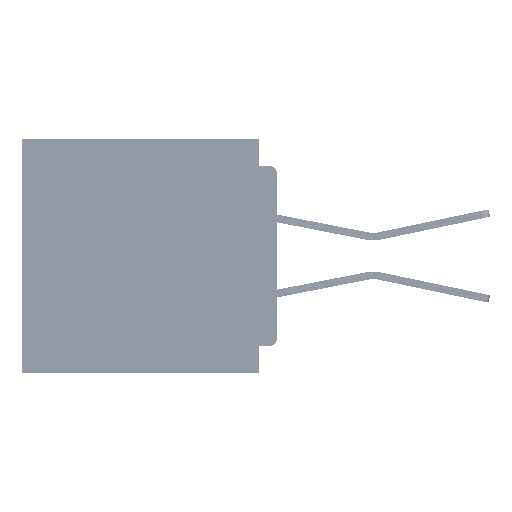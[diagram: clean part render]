
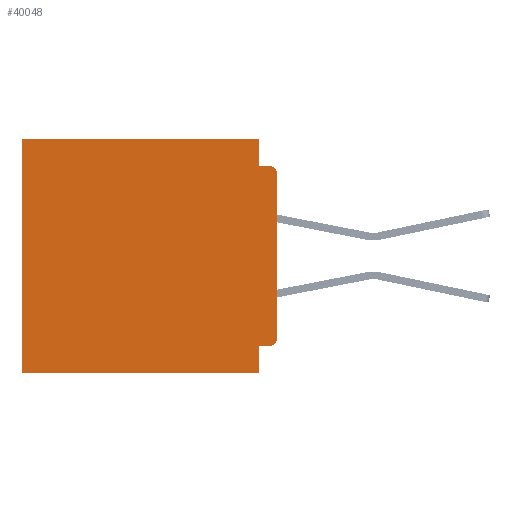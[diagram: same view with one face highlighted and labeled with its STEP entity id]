
A CAD part, left-side view. The second image highlights one B-rep face of the part: STEP entity #40048.
In plain terms, the highlighted planar face has unit normal (-1, 0, 0).
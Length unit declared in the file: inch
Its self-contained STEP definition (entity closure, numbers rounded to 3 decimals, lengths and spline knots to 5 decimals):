
#981 = VERTEX_POINT ( 'NONE', #3065 ) ;
#1917 = DIRECTION ( 'NONE',  ( 0., 1., 0. ) ) ;
#1973 = CARTESIAN_POINT ( 'NONE',  ( 0.3, 0.015, -0.34 ) ) ;
#2078 = ORIENTED_EDGE ( 'NONE', *, *, #9908, .T. ) ;
#2806 = VERTEX_POINT ( 'NONE', #18349 ) ;
#3065 = CARTESIAN_POINT ( 'NONE',  ( 0.3, 0.031, -0.045 ) ) ;
#3444 = EDGE_CURVE ( 'NONE', #34195, #33363, #9608, .T. ) ;
#4538 = CARTESIAN_POINT ( 'NONE',  ( 0.3, 0., -0.355 ) ) ;
#4986 = PLANE ( 'NONE',  #46262 ) ;
#5050 = CARTESIAN_POINT ( 'NONE',  ( 0.3, 0., -0.34 ) ) ;
#5322 = EDGE_CURVE ( 'NONE', #2806, #43426, #53814, .T. ) ;
#5660 = EDGE_CURVE ( 'NONE', #49036, #11780, #35707, .T. ) ;
#7135 = DIRECTION ( 'NONE',  ( 0., 0., -1. ) ) ;
#7487 = CARTESIAN_POINT ( 'NONE',  ( 0.3, 0.015, -0.06 ) ) ;
#8285 = ORIENTED_EDGE ( 'NONE', *, *, #41139, .T. ) ;
#8566 = VERTEX_POINT ( 'NONE', #5050 ) ;
#8852 = LINE ( 'NONE', #54566, #10474 ) ;
#8932 = EDGE_LOOP ( 'NONE', ( #15357, #13591, #13885, #32262, #8285, #56906, #37852, #56717, #35630, #2078 ) ) ;
#9608 = LINE ( 'NONE', #4538, #35096 ) ;
#9908 = EDGE_CURVE ( 'NONE', #34195, #8566, #17360, .T. ) ;
#10119 = CARTESIAN_POINT ( 'NONE',  ( 0.3, 0., -0.4 ) ) ;
#10474 = VECTOR ( 'NONE', #19109, 39.37008 ) ;
#10681 = CARTESIAN_POINT ( 'NONE',  ( 0.3, 0., -0.4 ) ) ;
#11780 = VERTEX_POINT ( 'NONE', #47954 ) ;
#12627 = DIRECTION ( 'NONE',  ( 0., 0., -1. ) ) ;
#13591 = ORIENTED_EDGE ( 'NONE', *, *, #5322, .T. ) ;
#13675 = VECTOR ( 'NONE', #29118, 39.37008 ) ;
#13885 = ORIENTED_EDGE ( 'NONE', *, *, #42511, .F. ) ;
#15235 = DIRECTION ( 'NONE',  ( 1., 0., 0. ) ) ;
#15357 = ORIENTED_EDGE ( 'NONE', *, *, #38884, .F. ) ;
#15817 = DIRECTION ( 'NONE',  ( 0., 0., -1. ) ) ;
#16157 = CARTESIAN_POINT ( 'NONE',  ( 0.3, 0.437, -0.4 ) ) ;
#17360 = CIRCLE ( 'NONE', #58397, 0.015 ) ;
#18349 = CARTESIAN_POINT ( 'NONE',  ( 0.3, 0., -0.06 ) ) ;
#19109 = DIRECTION ( 'NONE',  ( 0., 1., 0. ) ) ;
#20151 = CARTESIAN_POINT ( 'NONE',  ( 0.3, 0., -0.4 ) ) ;
#20365 = DIRECTION ( 'NONE',  ( 0., 0., -1. ) ) ;
#21446 = CARTESIAN_POINT ( 'NONE',  ( 0.3, 0.031, -0.355 ) ) ;
#21928 = CARTESIAN_POINT ( 'NONE',  ( 0.3, 0.015, -0.045 ) ) ;
#22177 = VECTOR ( 'NONE', #60693, 39.37008 ) ;
#24270 = DIRECTION ( 'NONE',  ( 0., -1., 0. ) ) ;
#24896 = CARTESIAN_POINT ( 'NONE',  ( 0.3, 0.031, -0.4 ) ) ;
#28815 = LINE ( 'NONE', #64538, #13675 ) ;
#28923 = AXIS2_PLACEMENT_3D ( 'NONE', #7487, #43062, #12627 ) ;
#29118 = DIRECTION ( 'NONE',  ( 0., 0., -1. ) ) ;
#32262 = ORIENTED_EDGE ( 'NONE', *, *, #35879, .F. ) ;
#33363 = VERTEX_POINT ( 'NONE', #21446 ) ;
#34195 = VERTEX_POINT ( 'NONE', #64536 ) ;
#34668 = VECTOR ( 'NONE', #15817, 39.37008 ) ;
#35096 = VECTOR ( 'NONE', #1917, 39.37008 ) ;
#35630 = ORIENTED_EDGE ( 'NONE', *, *, #3444, .F. ) ;
#35707 = LINE ( 'NONE', #20151, #22177 ) ;
#35879 = EDGE_CURVE ( 'NONE', #44845, #981, #36680, .T. ) ;
#36680 = LINE ( 'NONE', #60914, #46906 ) ;
#37616 = DIRECTION ( 'NONE',  ( -1., 0., 0. ) ) ;
#37772 = VECTOR ( 'NONE', #56708, 39.37008 ) ;
#37852 = ORIENTED_EDGE ( 'NONE', *, *, #5660, .F. ) ;
#38531 = FACE_OUTER_BOUND ( 'NONE', #8932, .T. ) ;
#38884 = EDGE_CURVE ( 'NONE', #2806, #8566, #48095, .T. ) ;
#40048 = ADVANCED_FACE ( 'NONE', ( #38531 ), #4986, .F. ) ;
#40275 = CARTESIAN_POINT ( 'NONE',  ( 0.3, 0.031, 0. ) ) ;
#41139 = EDGE_CURVE ( 'NONE', #44845, #52347, #8852, .T. ) ;
#42511 = EDGE_CURVE ( 'NONE', #981, #43426, #57204, .T. ) ;
#43062 = DIRECTION ( 'NONE',  ( -1., 0., 0. ) ) ;
#43426 = VERTEX_POINT ( 'NONE', #21928 ) ;
#43764 = VECTOR ( 'NONE', #24270, 39.37008 ) ;
#44845 = VERTEX_POINT ( 'NONE', #40275 ) ;
#45620 = CARTESIAN_POINT ( 'NONE',  ( 0.3, 0.437, 0. ) ) ;
#46262 = AXIS2_PLACEMENT_3D ( 'NONE', #10119, #15235, #50722 ) ;
#46906 = VECTOR ( 'NONE', #20365, 39.37008 ) ;
#47954 = CARTESIAN_POINT ( 'NONE',  ( 0.3, 0.437, -0.4 ) ) ;
#48095 = LINE ( 'NONE', #10681, #34668 ) ;
#49036 = VERTEX_POINT ( 'NONE', #24896 ) ;
#50722 = DIRECTION ( 'NONE',  ( 0., 0., -1. ) ) ;
#51179 = LINE ( 'NONE', #16157, #37772 ) ;
#52347 = VERTEX_POINT ( 'NONE', #45620 ) ;
#53814 = CIRCLE ( 'NONE', #28923, 0.015 ) ;
#54566 = CARTESIAN_POINT ( 'NONE',  ( 0.3, 0., 0. ) ) ;
#54622 = CARTESIAN_POINT ( 'NONE',  ( 0.3, 0., -0.045 ) ) ;
#56164 = EDGE_CURVE ( 'NONE', #52347, #11780, #51179, .T. ) ;
#56708 = DIRECTION ( 'NONE',  ( 0., 0., -1. ) ) ;
#56717 = ORIENTED_EDGE ( 'NONE', *, *, #64518, .F. ) ;
#56906 = ORIENTED_EDGE ( 'NONE', *, *, #56164, .T. ) ;
#57204 = LINE ( 'NONE', #54622, #43764 ) ;
#58397 = AXIS2_PLACEMENT_3D ( 'NONE', #1973, #37616, #7135 ) ;
#60693 = DIRECTION ( 'NONE',  ( 0., 1., 0. ) ) ;
#60914 = CARTESIAN_POINT ( 'NONE',  ( 0.3, 0.031, 0. ) ) ;
#64518 = EDGE_CURVE ( 'NONE', #33363, #49036, #28815, .T. ) ;
#64536 = CARTESIAN_POINT ( 'NONE',  ( 0.3, 0.015, -0.355 ) ) ;
#64538 = CARTESIAN_POINT ( 'NONE',  ( 0.3, 0.031, -0.4 ) ) ;
